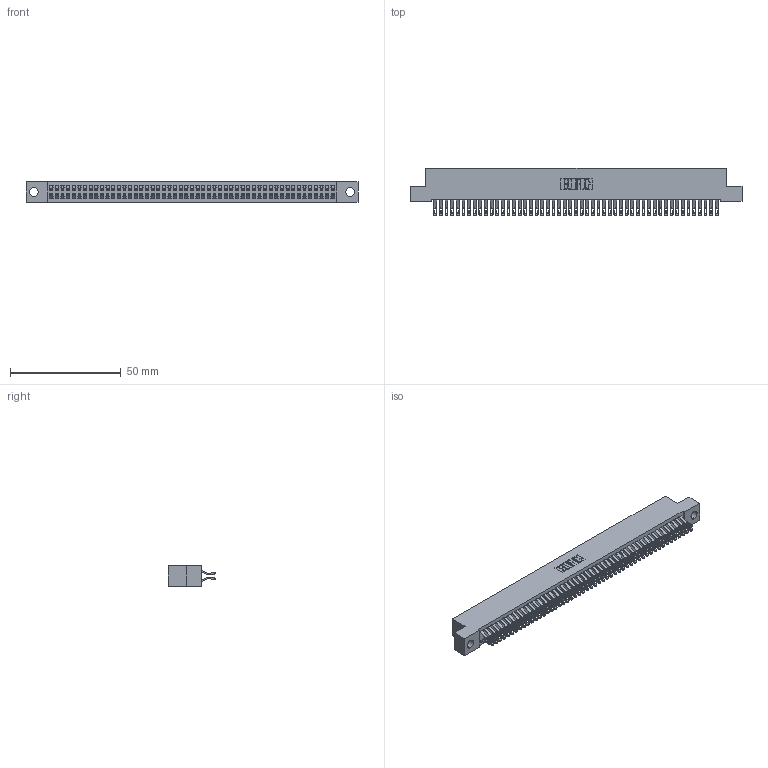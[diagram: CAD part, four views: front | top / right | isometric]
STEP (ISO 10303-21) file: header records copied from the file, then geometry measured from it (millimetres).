
FILE_DESCRIPTION (( 'STEP AP203' ), '1' );
FILE_NAME ('342-102-555-204.STEP', '2018-08-14T05:33:14', ( '' ), ( '' ), 'SwSTEP 2.0', 'SolidWorks 2016', '' );
FILE_SCHEMA (( 'CONFIG_CONTROL_DESIGN' ));
Length unit declared in the file: inch
Products named in the file (3): 342 Part_.156 TH; 345-292-001_555 Tail; 342-102-555-204
Assembly tree (103 placements, depth 2):
  342-102-555-204
    342 Part_.156 TH
    345-292-001_555 Tail  x102
Bounding box: 149.86 x 21.47 x 9.4 mm (x, y, z)
Volume: 13703.9 mm3; surface area: 23339.4 mm2
Topology: 103 solids, 103 shells, 6026 faces, 18965 edges, 12642 vertices
Faces by surface type: plane 3534, cylinder 2492
Entity records: 31843 total; most frequent: CARTESIAN_POINT 5300, ORIENTED_EDGE 5206, DIRECTION 4483, EDGE_CURVE 2603, VECTOR 2455, LINE 2455, VERTEX_POINT 1734, AXIS2_PLACEMENT_3D 1014
